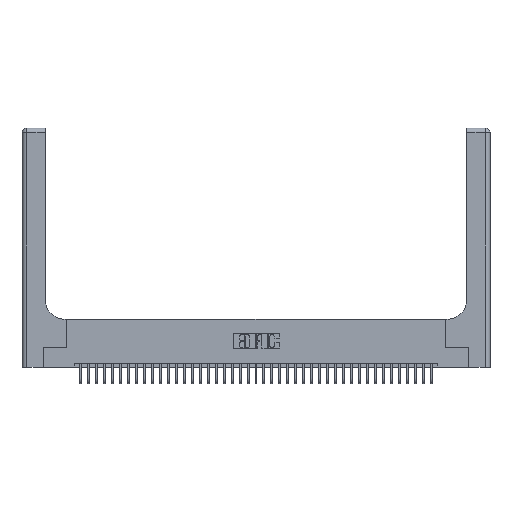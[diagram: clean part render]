
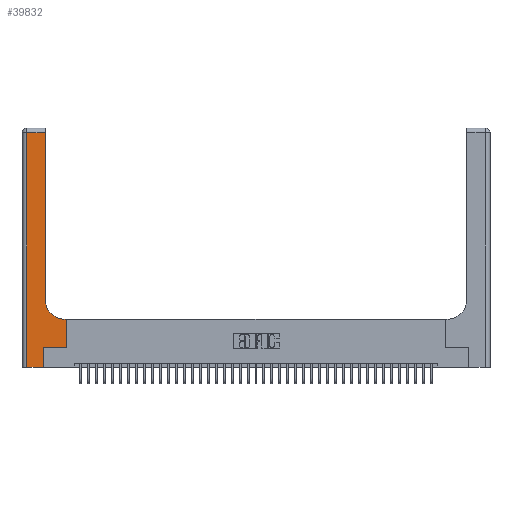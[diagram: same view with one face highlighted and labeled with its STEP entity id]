
A CAD part, top view. The second image highlights one B-rep face of the part: STEP entity #39832.
In plain terms, the highlighted planar face has unit normal (0, 0, 1).
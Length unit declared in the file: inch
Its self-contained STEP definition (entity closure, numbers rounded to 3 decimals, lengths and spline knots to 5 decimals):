
#332 = CARTESIAN_POINT ( 'NONE',  ( 0.269, 0.25, 0.37 ) ) ;
#611 = VECTOR ( 'NONE', #26065, 39.37008 ) ;
#1537 = ORIENTED_EDGE ( 'NONE', *, *, #37047, .T. ) ;
#1644 = LINE ( 'NONE', #332, #611 ) ;
#1855 = ORIENTED_EDGE ( 'NONE', *, *, #18004, .T. ) ;
#1973 = DIRECTION ( 'NONE',  ( -1., 0., 0. ) ) ;
#2178 = CARTESIAN_POINT ( 'NONE',  ( 0.269, 0., 0.37 ) ) ;
#2224 = VECTOR ( 'NONE', #31997, 39.37008 ) ;
#3697 = VERTEX_POINT ( 'NONE', #4087 ) ;
#4087 = CARTESIAN_POINT ( 'NONE',  ( 0.2915, 2.94, 0.37 ) ) ;
#5130 = CARTESIAN_POINT ( 'NONE',  ( 0.2915, 0.6, 0.37 ) ) ;
#5473 = DIRECTION ( 'NONE',  ( 0., 1., 0. ) ) ;
#5905 = FACE_OUTER_BOUND ( 'NONE', #16791, .T. ) ;
#5944 = VERTEX_POINT ( 'NONE', #5996 ) ;
#5974 = CARTESIAN_POINT ( 'NONE',  ( 0.5415, 0.6, 0.37 ) ) ;
#5996 = CARTESIAN_POINT ( 'NONE',  ( 0.06, 0., 0.37 ) ) ;
#6359 = ORIENTED_EDGE ( 'NONE', *, *, #27951, .T. ) ;
#7104 = EDGE_CURVE ( 'NONE', #22454, #8252, #13846, .T. ) ;
#8110 = ORIENTED_EDGE ( 'NONE', *, *, #34446, .T. ) ;
#8252 = VERTEX_POINT ( 'NONE', #31386 ) ;
#9268 = DIRECTION ( 'NONE',  ( 0., 0., -1. ) ) ;
#9997 = VERTEX_POINT ( 'NONE', #18729 ) ;
#11794 = VECTOR ( 'NONE', #12597, 39.37008 ) ;
#12597 = DIRECTION ( 'NONE',  ( 0., 1., 0. ) ) ;
#12838 = VECTOR ( 'NONE', #5473, 39.37008 ) ;
#13029 = VECTOR ( 'NONE', #27633, 39.37008 ) ;
#13846 = LINE ( 'NONE', #2178, #12838 ) ;
#14606 = DIRECTION ( 'NONE',  ( 0., 1., 0. ) ) ;
#14609 = VECTOR ( 'NONE', #1973, 39.37008 ) ;
#14700 = ORIENTED_EDGE ( 'NONE', *, *, #39612, .T. ) ;
#15055 = CARTESIAN_POINT ( 'NONE',  ( 0.06, 2.94, 0.37 ) ) ;
#15186 = CARTESIAN_POINT ( 'NONE',  ( 0., 3., 0.37 ) ) ;
#15578 = VERTEX_POINT ( 'NONE', #15055 ) ;
#16633 = CARTESIAN_POINT ( 'NONE',  ( 0.2915, 0.85, 0.37 ) ) ;
#16791 = EDGE_LOOP ( 'NONE', ( #24081, #24232, #8110, #14700, #21056, #1855, #35342, #1537, #6359 ) ) ;
#17325 = DIRECTION ( 'NONE',  ( 1., 0., 0. ) ) ;
#17553 = VERTEX_POINT ( 'NONE', #16633 ) ;
#18004 = EDGE_CURVE ( 'NONE', #8252, #9997, #1644, .T. ) ;
#18060 = VECTOR ( 'NONE', #14606, 39.37008 ) ;
#18278 = PLANE ( 'NONE',  #18601 ) ;
#18415 = DIRECTION ( 'NONE',  ( -1., 0., 0. ) ) ;
#18601 = AXIS2_PLACEMENT_3D ( 'NONE', #15186, #37744, #18415 ) ;
#18729 = CARTESIAN_POINT ( 'NONE',  ( 0.5585, 0.25, 0.37 ) ) ;
#19043 = CARTESIAN_POINT ( 'NONE',  ( 0.5585, 0.25, 0.37 ) ) ;
#19709 = EDGE_CURVE ( 'NONE', #3697, #15578, #38722, .T. ) ;
#20335 = LINE ( 'NONE', #19043, #11794 ) ;
#21056 = ORIENTED_EDGE ( 'NONE', *, *, #7104, .T. ) ;
#21221 = CARTESIAN_POINT ( 'NONE',  ( 0., 2.94, 0.37 ) ) ;
#21478 = CIRCLE ( 'NONE', #32353, 0.25 ) ;
#22454 = VERTEX_POINT ( 'NONE', #28860 ) ;
#23195 = EDGE_CURVE ( 'NONE', #9997, #30520, #20335, .T. ) ;
#24081 = ORIENTED_EDGE ( 'NONE', *, *, #31833, .T. ) ;
#24232 = ORIENTED_EDGE ( 'NONE', *, *, #19709, .T. ) ;
#26065 = DIRECTION ( 'NONE',  ( 1., 0., 0. ) ) ;
#27633 = DIRECTION ( 'NONE',  ( -1., 0., 0. ) ) ;
#27864 = LINE ( 'NONE', #35267, #2224 ) ;
#27951 = EDGE_CURVE ( 'NONE', #37186, #17553, #21478, .T. ) ;
#28448 = CARTESIAN_POINT ( 'NONE',  ( 0.5415, 0.85, 0.37 ) ) ;
#28860 = CARTESIAN_POINT ( 'NONE',  ( 0.269, 0., 0.37 ) ) ;
#30520 = VERTEX_POINT ( 'NONE', #41570 ) ;
#30773 = CARTESIAN_POINT ( 'NONE',  ( 0.2915, 3., 0.37 ) ) ;
#31033 = LINE ( 'NONE', #33384, #38627 ) ;
#31386 = CARTESIAN_POINT ( 'NONE',  ( 0.269, 0.25, 0.37 ) ) ;
#31729 = DIRECTION ( 'NONE',  ( 1., 0., 0. ) ) ;
#31833 = EDGE_CURVE ( 'NONE', #17553, #3697, #35217, .T. ) ;
#31997 = DIRECTION ( 'NONE',  ( 0., -1., 0. ) ) ;
#32353 = AXIS2_PLACEMENT_3D ( 'NONE', #28448, #9268, #31729 ) ;
#32751 = LINE ( 'NONE', #5130, #14609 ) ;
#33384 = CARTESIAN_POINT ( 'NONE',  ( 0., 0., 0.37 ) ) ;
#34446 = EDGE_CURVE ( 'NONE', #15578, #5944, #27864, .T. ) ;
#35217 = LINE ( 'NONE', #30773, #18060 ) ;
#35267 = CARTESIAN_POINT ( 'NONE',  ( 0.06, 3., 0.37 ) ) ;
#35342 = ORIENTED_EDGE ( 'NONE', *, *, #23195, .T. ) ;
#37047 = EDGE_CURVE ( 'NONE', #30520, #37186, #32751, .T. ) ;
#37186 = VERTEX_POINT ( 'NONE', #5974 ) ;
#37744 = DIRECTION ( 'NONE',  ( 0., 0., -1. ) ) ;
#38627 = VECTOR ( 'NONE', #17325, 39.37008 ) ;
#38722 = LINE ( 'NONE', #21221, #13029 ) ;
#39612 = EDGE_CURVE ( 'NONE', #5944, #22454, #31033, .T. ) ;
#39832 = ADVANCED_FACE ( 'NONE', ( #5905 ), #18278, .F. ) ;
#41570 = CARTESIAN_POINT ( 'NONE',  ( 0.5585, 0.6, 0.37 ) ) ;
